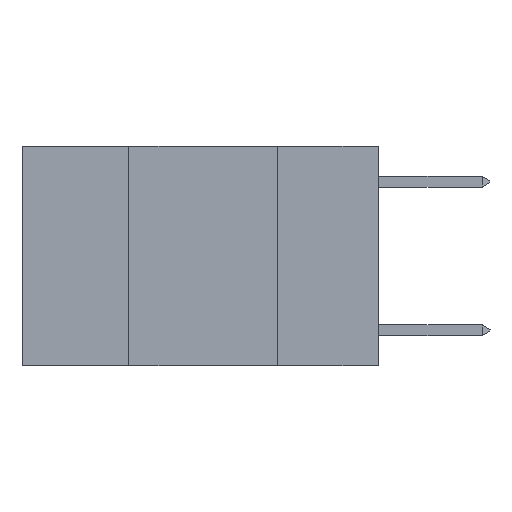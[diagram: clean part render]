
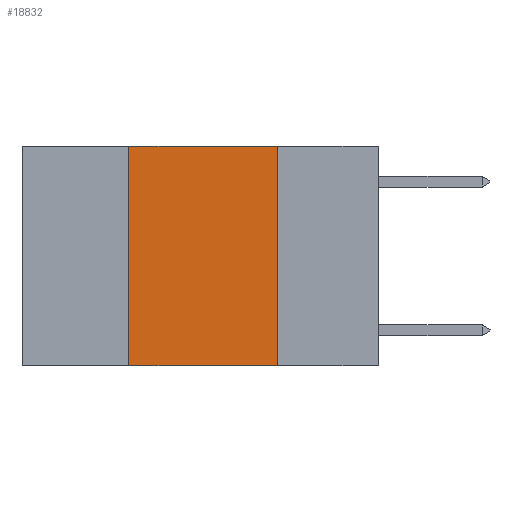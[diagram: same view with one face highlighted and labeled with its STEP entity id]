
A CAD part, left-side view. The second image highlights one B-rep face of the part: STEP entity #18832.
In plain terms, the highlighted planar face has unit normal (-1, 0, 0).
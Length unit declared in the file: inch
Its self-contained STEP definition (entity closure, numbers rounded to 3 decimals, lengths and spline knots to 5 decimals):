
#1305 = VECTOR ( 'NONE', #12941, 39.37008 ) ;
#1668 = EDGE_CURVE ( 'NONE', #10250, #4302, #7699, .T. ) ;
#2392 = LINE ( 'NONE', #7305, #6071 ) ;
#2544 = EDGE_CURVE ( 'NONE', #11804, #10250, #10009, .T. ) ;
#3412 = CARTESIAN_POINT ( 'NONE',  ( 0., 0.6, 0. ) ) ;
#3454 = CARTESIAN_POINT ( 'NONE',  ( 0., 0.42, 0. ) ) ;
#3478 = DIRECTION ( 'NONE',  ( 0., 0., 1. ) ) ;
#4302 = VERTEX_POINT ( 'NONE', #12835 ) ;
#4331 = CARTESIAN_POINT ( 'NONE',  ( 0., 0.17, -0.37 ) ) ;
#4994 = DIRECTION ( 'NONE',  ( 1., 0., 0. ) ) ;
#5165 = LINE ( 'NONE', #19110, #12019 ) ;
#6071 = VECTOR ( 'NONE', #7032, 39.37008 ) ;
#7032 = DIRECTION ( 'NONE',  ( 0., 0., -1. ) ) ;
#7305 = CARTESIAN_POINT ( 'NONE',  ( 0., 0.17, 0. ) ) ;
#7699 = LINE ( 'NONE', #12737, #1305 ) ;
#9035 = CARTESIAN_POINT ( 'NONE',  ( 0., 0.42, -0.37 ) ) ;
#9270 = FACE_OUTER_BOUND ( 'NONE', #16449, .T. ) ;
#9372 = EDGE_CURVE ( 'NONE', #4302, #14142, #2392, .T. ) ;
#10009 = LINE ( 'NONE', #3454, #17663 ) ;
#10236 = CARTESIAN_POINT ( 'NONE',  ( 0., 0.42, 0. ) ) ;
#10250 = VERTEX_POINT ( 'NONE', #10236 ) ;
#11600 = DIRECTION ( 'NONE',  ( 0., -1., 0. ) ) ;
#11804 = VERTEX_POINT ( 'NONE', #9035 ) ;
#12019 = VECTOR ( 'NONE', #11600, 39.37008 ) ;
#12737 = CARTESIAN_POINT ( 'NONE',  ( 0., 0.6, 0. ) ) ;
#12794 = PLANE ( 'NONE',  #18481 ) ;
#12835 = CARTESIAN_POINT ( 'NONE',  ( 0., 0.17, 0. ) ) ;
#12941 = DIRECTION ( 'NONE',  ( 0., -1., 0. ) ) ;
#13887 = EDGE_CURVE ( 'NONE', #11804, #14142, #5165, .T. ) ;
#14142 = VERTEX_POINT ( 'NONE', #4331 ) ;
#15830 = DIRECTION ( 'NONE',  ( 0., 0., -1. ) ) ;
#16449 = EDGE_LOOP ( 'NONE', ( #16659, #16732, #16957, #16971 ) ) ;
#16659 = ORIENTED_EDGE ( 'NONE', *, *, #9372, .F. ) ;
#16732 = ORIENTED_EDGE ( 'NONE', *, *, #1668, .F. ) ;
#16957 = ORIENTED_EDGE ( 'NONE', *, *, #2544, .F. ) ;
#16971 = ORIENTED_EDGE ( 'NONE', *, *, #13887, .T. ) ;
#17663 = VECTOR ( 'NONE', #3478, 39.37008 ) ;
#18481 = AXIS2_PLACEMENT_3D ( 'NONE', #3412, #4994, #15830 ) ;
#18832 = ADVANCED_FACE ( 'NONE', ( #9270 ), #12794, .F. ) ;
#19110 = CARTESIAN_POINT ( 'NONE',  ( 0., 0.6, -0.37 ) ) ;
